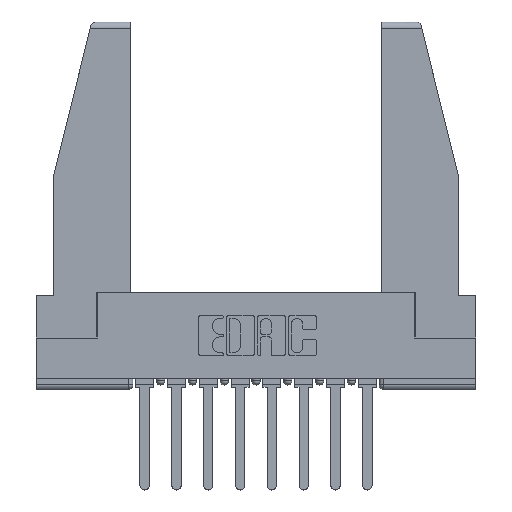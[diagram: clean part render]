
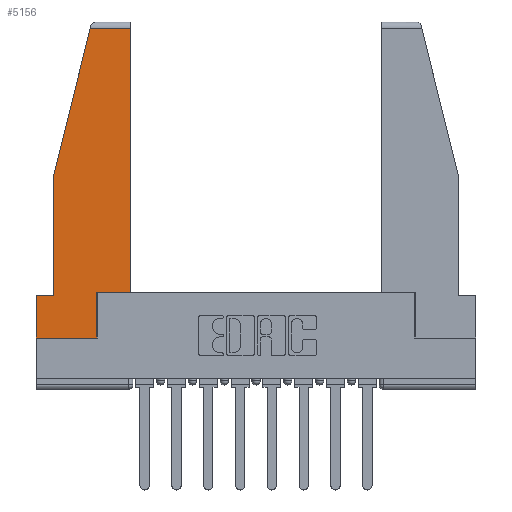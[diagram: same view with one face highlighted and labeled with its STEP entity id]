
A CAD part, top view. The second image highlights one B-rep face of the part: STEP entity #5156.
In plain terms, the highlighted planar face has unit normal (0, 0, 1).
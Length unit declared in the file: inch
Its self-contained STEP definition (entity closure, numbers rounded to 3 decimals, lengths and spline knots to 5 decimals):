
#313 = CARTESIAN_POINT ( 'NONE',  ( 0.2636, 1.52, 0. ) ) ;
#503 = VERTEX_POINT ( 'NONE', #9862 ) ;
#1126 = PLANE ( 'NONE',  #2101 ) ;
#1164 = CARTESIAN_POINT ( 'NONE',  ( 0., 1.52, 0. ) ) ;
#1304 = CARTESIAN_POINT ( 'NONE',  ( 0., 0.21, 0. ) ) ;
#1425 = EDGE_CURVE ( 'NONE', #8603, #5550, #7079, .T. ) ;
#2047 = DIRECTION ( 'NONE',  ( -0.239, -0.971, 0. ) ) ;
#2101 = AXIS2_PLACEMENT_3D ( 'NONE', #13200, #6662, #10362 ) ;
#2496 = CARTESIAN_POINT ( 'NONE',  ( 0., 0., 0. ) ) ;
#2863 = ORIENTED_EDGE ( 'NONE', *, *, #2887, .T. ) ;
#2887 = EDGE_CURVE ( 'NONE', #503, #5566, #4536, .T. ) ;
#3104 = VECTOR ( 'NONE', #6108, 39.37008 ) ;
#3662 = CARTESIAN_POINT ( 'NONE',  ( 0.461, 0.223, 0. ) ) ;
#3726 = VECTOR ( 'NONE', #10114, 39.37008 ) ;
#4123 = EDGE_CURVE ( 'NONE', #5944, #503, #9423, .T. ) ;
#4435 = VECTOR ( 'NONE', #5777, 39.37008 ) ;
#4536 = LINE ( 'NONE', #1164, #3726 ) ;
#4565 = ORIENTED_EDGE ( 'NONE', *, *, #4123, .T. ) ;
#4898 = CARTESIAN_POINT ( 'NONE',  ( 0.297, 0., 0. ) ) ;
#5156 = ADVANCED_FACE ( 'NONE', ( #11070 ), #1126, .T. ) ;
#5234 = ORIENTED_EDGE ( 'NONE', *, *, #9366, .T. ) ;
#5412 = LINE ( 'NONE', #6447, #10912 ) ;
#5445 = EDGE_CURVE ( 'NONE', #10705, #5767, #11120, .T. ) ;
#5550 = VERTEX_POINT ( 'NONE', #11611 ) ;
#5562 = CARTESIAN_POINT ( 'NONE',  ( 0., 0., 0. ) ) ;
#5566 = VERTEX_POINT ( 'NONE', #313 ) ;
#5767 = VERTEX_POINT ( 'NONE', #1304 ) ;
#5777 = DIRECTION ( 'NONE',  ( -1., 0., 0. ) ) ;
#5944 = VERTEX_POINT ( 'NONE', #3662 ) ;
#6108 = DIRECTION ( 'NONE',  ( 1., 0., 0. ) ) ;
#6383 = EDGE_CURVE ( 'NONE', #5566, #9222, #5412, .T. ) ;
#6447 = CARTESIAN_POINT ( 'NONE',  ( 0.271, 1.55, 0. ) ) ;
#6662 = DIRECTION ( 'NONE',  ( 0., 0., 1. ) ) ;
#6874 = ORIENTED_EDGE ( 'NONE', *, *, #11381, .T. ) ;
#7079 = LINE ( 'NONE', #4898, #10342 ) ;
#7136 = LINE ( 'NONE', #12589, #7871 ) ;
#7139 = EDGE_CURVE ( 'NONE', #9222, #10705, #7136, .T. ) ;
#7325 = DIRECTION ( 'NONE',  ( 0., 1., 0. ) ) ;
#7519 = CARTESIAN_POINT ( 'NONE',  ( 0., 0.21, 0. ) ) ;
#7574 = ORIENTED_EDGE ( 'NONE', *, *, #10319, .T. ) ;
#7871 = VECTOR ( 'NONE', #13603, 39.37008 ) ;
#8053 = ORIENTED_EDGE ( 'NONE', *, *, #7139, .T. ) ;
#8162 = VECTOR ( 'NONE', #13340, 39.37008 ) ;
#8377 = CARTESIAN_POINT ( 'NONE',  ( 0.086, 0.8, 0. ) ) ;
#8449 = VECTOR ( 'NONE', #7325, 39.37008 ) ;
#8603 = VERTEX_POINT ( 'NONE', #13299 ) ;
#8977 = LINE ( 'NONE', #5562, #8162 ) ;
#8980 = ORIENTED_EDGE ( 'NONE', *, *, #5445, .T. ) ;
#9222 = VERTEX_POINT ( 'NONE', #8377 ) ;
#9293 = LINE ( 'NONE', #13657, #3104 ) ;
#9366 = EDGE_CURVE ( 'NONE', #5550, #5944, #9293, .T. ) ;
#9423 = LINE ( 'NONE', #10712, #8449 ) ;
#9677 = VERTEX_POINT ( 'NONE', #2496 ) ;
#9862 = CARTESIAN_POINT ( 'NONE',  ( 0.461, 1.52, 0. ) ) ;
#9907 = CARTESIAN_POINT ( 'NONE',  ( 0., 0.21, 0. ) ) ;
#10114 = DIRECTION ( 'NONE',  ( -1., 0., 0. ) ) ;
#10319 = EDGE_CURVE ( 'NONE', #5767, #9677, #13989, .T. ) ;
#10342 = VECTOR ( 'NONE', #13615, 39.37008 ) ;
#10362 = DIRECTION ( 'NONE',  ( 1., 0., 0. ) ) ;
#10508 = VECTOR ( 'NONE', #11693, 39.37008 ) ;
#10705 = VERTEX_POINT ( 'NONE', #11533 ) ;
#10712 = CARTESIAN_POINT ( 'NONE',  ( 0.461, 0.223, 0. ) ) ;
#10912 = VECTOR ( 'NONE', #2047, 39.37008 ) ;
#11070 = FACE_OUTER_BOUND ( 'NONE', #13706, .T. ) ;
#11120 = LINE ( 'NONE', #9907, #4435 ) ;
#11381 = EDGE_CURVE ( 'NONE', #9677, #8603, #8977, .T. ) ;
#11533 = CARTESIAN_POINT ( 'NONE',  ( 0.086, 0.21, 0. ) ) ;
#11611 = CARTESIAN_POINT ( 'NONE',  ( 0.297, 0.223, 0. ) ) ;
#11693 = DIRECTION ( 'NONE',  ( 0., -1., 0. ) ) ;
#12490 = ORIENTED_EDGE ( 'NONE', *, *, #1425, .T. ) ;
#12589 = CARTESIAN_POINT ( 'NONE',  ( 0.086, 0.8, 0. ) ) ;
#13200 = CARTESIAN_POINT ( 'NONE',  ( 0., 0., 0. ) ) ;
#13299 = CARTESIAN_POINT ( 'NONE',  ( 0.297, 0., 0. ) ) ;
#13340 = DIRECTION ( 'NONE',  ( 1., 0., 0. ) ) ;
#13515 = ORIENTED_EDGE ( 'NONE', *, *, #6383, .T. ) ;
#13603 = DIRECTION ( 'NONE',  ( 0., -1., 0. ) ) ;
#13615 = DIRECTION ( 'NONE',  ( 0., 1., 0. ) ) ;
#13657 = CARTESIAN_POINT ( 'NONE',  ( 0.297, 0.223, 0. ) ) ;
#13706 = EDGE_LOOP ( 'NONE', ( #4565, #2863, #13515, #8053, #8980, #7574, #6874, #12490, #5234 ) ) ;
#13989 = LINE ( 'NONE', #7519, #10508 ) ;
